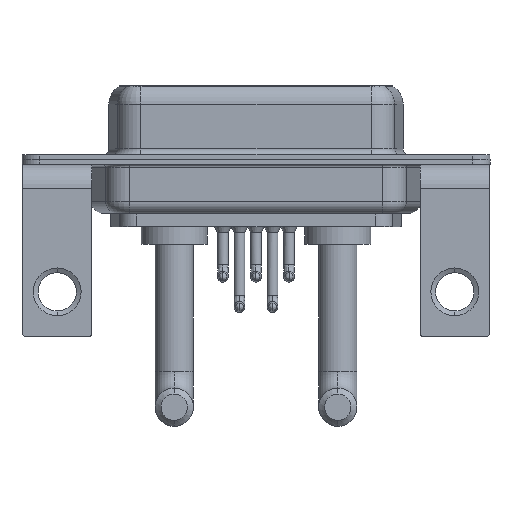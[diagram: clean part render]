
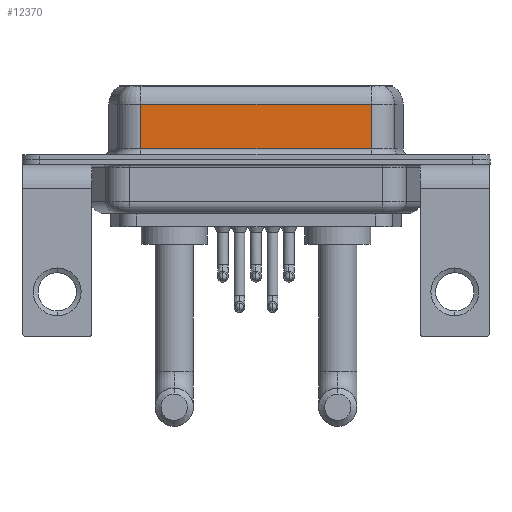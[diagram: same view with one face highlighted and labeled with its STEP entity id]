
A CAD part, front view. The second image highlights one B-rep face of the part: STEP entity #12370.
In plain terms, the highlighted planar face has unit normal (0, -1, 0).
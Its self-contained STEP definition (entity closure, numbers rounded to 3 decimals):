
#597 = DIRECTION ( 'NONE',  ( 0., 1., 0. ) ) ;
#676 = VERTEX_POINT ( 'NONE', #14993 ) ;
#2491 = DIRECTION ( 'NONE',  ( 1., 0., 0. ) ) ;
#2546 = AXIS2_PLACEMENT_3D ( 'NONE', #6147, #597, #16949 ) ;
#3067 = ORIENTED_EDGE ( 'NONE', *, *, #17184, .T. ) ;
#3089 = CARTESIAN_POINT ( 'NONE',  ( 7.013, -3.95, 4.65 ) ) ;
#3179 = VERTEX_POINT ( 'NONE', #11715 ) ;
#3496 = VERTEX_POINT ( 'NONE', #7141 ) ;
#3577 = LINE ( 'NONE', #16079, #17091 ) ;
#3604 = ORIENTED_EDGE ( 'NONE', *, *, #12051, .T. ) ;
#5095 = VECTOR ( 'NONE', #14040, 1000. ) ;
#5367 = VERTEX_POINT ( 'NONE', #3089 ) ;
#6147 = CARTESIAN_POINT ( 'NONE',  ( 26.287, -3.95, 6.4 ) ) ;
#7141 = CARTESIAN_POINT ( 'NONE',  ( 7.013, -3.95, 0.9 ) ) ;
#7612 = LINE ( 'NONE', #17250, #8234 ) ;
#8234 = VECTOR ( 'NONE', #11719, 1000. ) ;
#9964 = EDGE_CURVE ( 'NONE', #676, #5367, #11362, .T. ) ;
#10080 = VECTOR ( 'NONE', #12055, 1000. ) ;
#10089 = PLANE ( 'NONE',  #2546 ) ;
#10134 = EDGE_CURVE ( 'NONE', #676, #3179, #7612, .T. ) ;
#10475 = EDGE_LOOP ( 'NONE', ( #14229, #10728, #3067, #3604 ) ) ;
#10728 = ORIENTED_EDGE ( 'NONE', *, *, #9964, .T. ) ;
#11362 = LINE ( 'NONE', #17071, #5095 ) ;
#11715 = CARTESIAN_POINT ( 'NONE',  ( 26.287, -3.95, 0.9 ) ) ;
#11719 = DIRECTION ( 'NONE',  ( 0., 0., -1. ) ) ;
#12051 = EDGE_CURVE ( 'NONE', #3496, #3179, #3577, .T. ) ;
#12055 = DIRECTION ( 'NONE',  ( 0., 0., -1. ) ) ;
#12370 = ADVANCED_FACE ( 'NONE', ( #12842 ), #10089, .F. ) ;
#12842 = FACE_OUTER_BOUND ( 'NONE', #10475, .T. ) ;
#14040 = DIRECTION ( 'NONE',  ( -1., 0., 0. ) ) ;
#14229 = ORIENTED_EDGE ( 'NONE', *, *, #10134, .F. ) ;
#14993 = CARTESIAN_POINT ( 'NONE',  ( 26.287, -3.95, 4.65 ) ) ;
#16079 = CARTESIAN_POINT ( 'NONE',  ( 26.287, -3.95, 0.9 ) ) ;
#16257 = CARTESIAN_POINT ( 'NONE',  ( 7.013, -3.95, 6.4 ) ) ;
#16949 = DIRECTION ( 'NONE',  ( 0., 0., 1. ) ) ;
#17071 = CARTESIAN_POINT ( 'NONE',  ( 26.287, -3.95, 4.65 ) ) ;
#17091 = VECTOR ( 'NONE', #2491, 1000. ) ;
#17184 = EDGE_CURVE ( 'NONE', #5367, #3496, #17309, .T. ) ;
#17250 = CARTESIAN_POINT ( 'NONE',  ( 26.287, -3.95, 6.4 ) ) ;
#17309 = LINE ( 'NONE', #16257, #10080 ) ;
